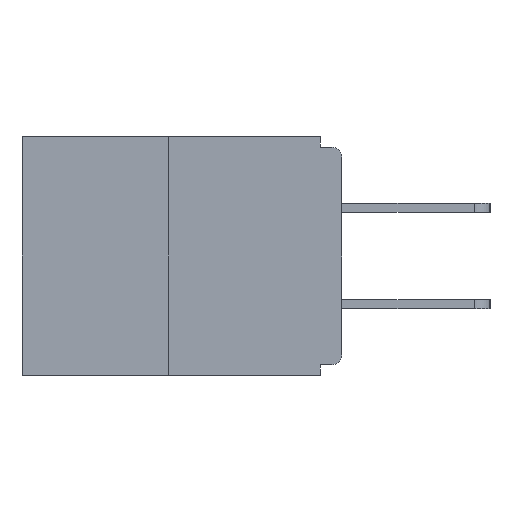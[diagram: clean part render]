
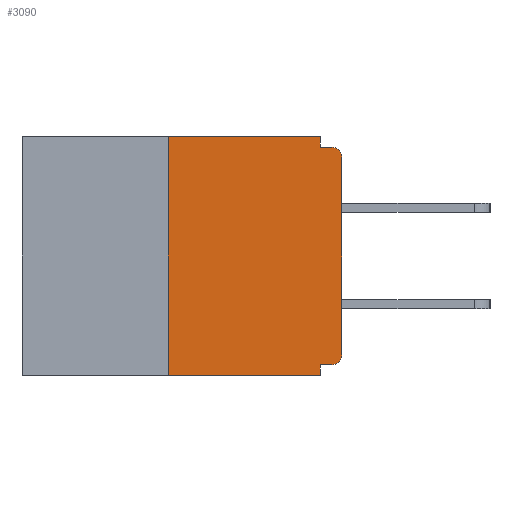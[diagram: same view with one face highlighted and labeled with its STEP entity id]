
A CAD part, left-side view. The second image highlights one B-rep face of the part: STEP entity #3090.
In plain terms, the highlighted planar face has unit normal (-1, 0, 0).
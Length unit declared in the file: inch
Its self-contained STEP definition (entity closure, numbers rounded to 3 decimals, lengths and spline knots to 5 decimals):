
#136 = DIRECTION ( 'NONE',  ( 0., 0., 1. ) ) ;
#208 = CARTESIAN_POINT ( 'NONE',  ( 0., 0.031, 0. ) ) ;
#305 = CARTESIAN_POINT ( 'NONE',  ( 0., 0.031, -0.343 ) ) ;
#514 = ORIENTED_EDGE ( 'NONE', *, *, #10167, .F. ) ;
#564 = DIRECTION ( 'NONE',  ( 1., 0., 0. ) ) ;
#646 = VERTEX_POINT ( 'NONE', #6234 ) ;
#682 = VECTOR ( 'NONE', #10117, 39.37008 ) ;
#1086 = DIRECTION ( 'NONE',  ( 0., -1., 0. ) ) ;
#1187 = EDGE_CURVE ( 'NONE', #1358, #7956, #4750, .T. ) ;
#1358 = VERTEX_POINT ( 'NONE', #16208 ) ;
#1682 = VERTEX_POINT ( 'NONE', #11228 ) ;
#1771 = ORIENTED_EDGE ( 'NONE', *, *, #8317, .T. ) ;
#1890 = CARTESIAN_POINT ( 'NONE',  ( 0., 0.46, 0. ) ) ;
#1945 = ORIENTED_EDGE ( 'NONE', *, *, #10455, .F. ) ;
#2515 = DIRECTION ( 'NONE',  ( 0., -1., 0. ) ) ;
#2941 = DIRECTION ( 'NONE',  ( 0., 0., 1. ) ) ;
#3090 = ADVANCED_FACE ( 'NONE', ( #17336 ), #11790, .F. ) ;
#3283 = CARTESIAN_POINT ( 'NONE',  ( 0., 0.015, -0.328 ) ) ;
#3566 = VECTOR ( 'NONE', #15756, 39.37008 ) ;
#3730 = EDGE_CURVE ( 'NONE', #1682, #13988, #6205, .T. ) ;
#3982 = CIRCLE ( 'NONE', #15765, 0.015 ) ;
#4744 = CARTESIAN_POINT ( 'NONE',  ( 0., 0.015, -0.313 ) ) ;
#4750 = LINE ( 'NONE', #9577, #15226 ) ;
#5028 = DIRECTION ( 'NONE',  ( 0., -1., 0. ) ) ;
#5059 = EDGE_CURVE ( 'NONE', #13958, #7329, #3982, .T. ) ;
#5289 = ORIENTED_EDGE ( 'NONE', *, *, #3730, .T. ) ;
#5433 = ORIENTED_EDGE ( 'NONE', *, *, #1187, .T. ) ;
#5855 = AXIS2_PLACEMENT_3D ( 'NONE', #1890, #564, #12111 ) ;
#6205 = CIRCLE ( 'NONE', #6945, 0.015 ) ;
#6231 = CARTESIAN_POINT ( 'NONE',  ( 0., 0.031, 0. ) ) ;
#6234 = CARTESIAN_POINT ( 'NONE',  ( 0., 0.25, 0. ) ) ;
#6945 = AXIS2_PLACEMENT_3D ( 'NONE', #15512, #10489, #16438 ) ;
#7135 = VERTEX_POINT ( 'NONE', #11344 ) ;
#7191 = CARTESIAN_POINT ( 'NONE',  ( 0., 0.031, -0.343 ) ) ;
#7248 = CARTESIAN_POINT ( 'NONE',  ( 0., 0., 0. ) ) ;
#7329 = VERTEX_POINT ( 'NONE', #9565 ) ;
#7597 = LINE ( 'NONE', #10996, #15180 ) ;
#7709 = VECTOR ( 'NONE', #5028, 39.37008 ) ;
#7956 = VERTEX_POINT ( 'NONE', #305 ) ;
#8317 = EDGE_CURVE ( 'NONE', #7329, #1682, #12161, .T. ) ;
#9400 = VERTEX_POINT ( 'NONE', #6231 ) ;
#9520 = LINE ( 'NONE', #13553, #7709 ) ;
#9565 = CARTESIAN_POINT ( 'NONE',  ( 0., 0., -0.313 ) ) ;
#9577 = CARTESIAN_POINT ( 'NONE',  ( 0., 0.46, -0.343 ) ) ;
#10117 = DIRECTION ( 'NONE',  ( 0., 0., -1. ) ) ;
#10167 = EDGE_CURVE ( 'NONE', #9400, #14073, #15395, .T. ) ;
#10229 = DIRECTION ( 'NONE',  ( 0., 0., -1. ) ) ;
#10438 = ORIENTED_EDGE ( 'NONE', *, *, #12164, .F. ) ;
#10455 = EDGE_CURVE ( 'NONE', #14073, #13988, #9520, .T. ) ;
#10489 = DIRECTION ( 'NONE',  ( -1., 0., 0. ) ) ;
#10698 = EDGE_CURVE ( 'NONE', #7135, #7956, #13387, .T. ) ;
#10996 = CARTESIAN_POINT ( 'NONE',  ( 0., 0., -0.328 ) ) ;
#11228 = CARTESIAN_POINT ( 'NONE',  ( 0., 0., -0.03 ) ) ;
#11344 = CARTESIAN_POINT ( 'NONE',  ( 0., 0.031, -0.328 ) ) ;
#11755 = LINE ( 'NONE', #17247, #12881 ) ;
#11790 = PLANE ( 'NONE',  #5855 ) ;
#12111 = DIRECTION ( 'NONE',  ( 0., 0., -1. ) ) ;
#12161 = LINE ( 'NONE', #7248, #12594 ) ;
#12164 = EDGE_CURVE ( 'NONE', #1358, #646, #11755, .T. ) ;
#12594 = VECTOR ( 'NONE', #136, 39.37008 ) ;
#12881 = VECTOR ( 'NONE', #2941, 39.37008 ) ;
#13387 = LINE ( 'NONE', #7191, #3566 ) ;
#13553 = CARTESIAN_POINT ( 'NONE',  ( 0., 0., -0.015 ) ) ;
#13958 = VERTEX_POINT ( 'NONE', #3283 ) ;
#13988 = VERTEX_POINT ( 'NONE', #16029 ) ;
#14073 = VERTEX_POINT ( 'NONE', #15320 ) ;
#14718 = DIRECTION ( 'NONE',  ( -1., 0., 0. ) ) ;
#15180 = VECTOR ( 'NONE', #18194, 39.37008 ) ;
#15226 = VECTOR ( 'NONE', #2515, 39.37008 ) ;
#15320 = CARTESIAN_POINT ( 'NONE',  ( 0., 0.031, -0.015 ) ) ;
#15395 = LINE ( 'NONE', #208, #682 ) ;
#15512 = CARTESIAN_POINT ( 'NONE',  ( 0., 0.015, -0.03 ) ) ;
#15712 = EDGE_LOOP ( 'NONE', ( #17939, #10438, #5433, #17200, #15890, #17654, #1771, #5289, #1945, #514 ) ) ;
#15756 = DIRECTION ( 'NONE',  ( 0., 0., -1. ) ) ;
#15765 = AXIS2_PLACEMENT_3D ( 'NONE', #4744, #14718, #10229 ) ;
#15890 = ORIENTED_EDGE ( 'NONE', *, *, #16361, .F. ) ;
#16029 = CARTESIAN_POINT ( 'NONE',  ( 0., 0.015, -0.015 ) ) ;
#16111 = LINE ( 'NONE', #16662, #16561 ) ;
#16208 = CARTESIAN_POINT ( 'NONE',  ( 0., 0.25, -0.343 ) ) ;
#16361 = EDGE_CURVE ( 'NONE', #13958, #7135, #7597, .T. ) ;
#16438 = DIRECTION ( 'NONE',  ( 0., 0., -1. ) ) ;
#16561 = VECTOR ( 'NONE', #1086, 39.37008 ) ;
#16662 = CARTESIAN_POINT ( 'NONE',  ( 0., 0.46, 0. ) ) ;
#17028 = EDGE_CURVE ( 'NONE', #646, #9400, #16111, .T. ) ;
#17200 = ORIENTED_EDGE ( 'NONE', *, *, #10698, .F. ) ;
#17247 = CARTESIAN_POINT ( 'NONE',  ( 0., 0.25, 0. ) ) ;
#17336 = FACE_OUTER_BOUND ( 'NONE', #15712, .T. ) ;
#17654 = ORIENTED_EDGE ( 'NONE', *, *, #5059, .T. ) ;
#17939 = ORIENTED_EDGE ( 'NONE', *, *, #17028, .F. ) ;
#18194 = DIRECTION ( 'NONE',  ( 0., 1., 0. ) ) ;
